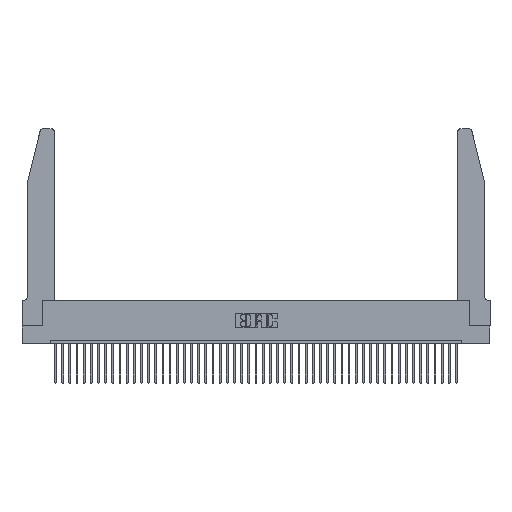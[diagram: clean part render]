
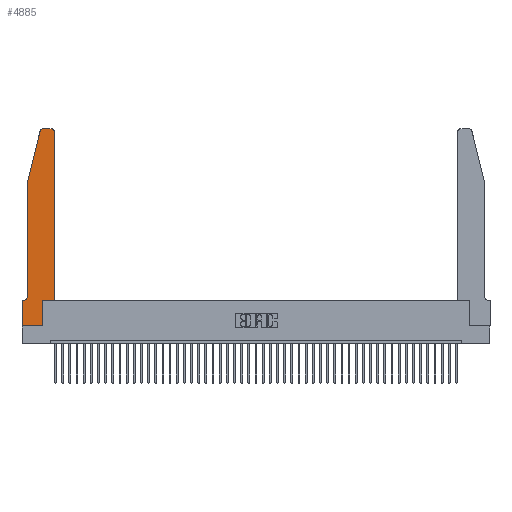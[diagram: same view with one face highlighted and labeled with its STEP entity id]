
A CAD part, top view. The second image highlights one B-rep face of the part: STEP entity #4885.
In plain terms, the highlighted planar face has unit normal (0, 0, 1).
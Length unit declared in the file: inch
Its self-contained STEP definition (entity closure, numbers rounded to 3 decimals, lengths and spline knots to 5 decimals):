
#571 = ORIENTED_EDGE ( 'NONE', *, *, #3788, .T. ) ;
#582 = CARTESIAN_POINT ( 'NONE',  ( 0.4205, 2.72, 0.37 ) ) ;
#734 = VECTOR ( 'NONE', #34522, 39.37008 ) ;
#787 = EDGE_CURVE ( 'NONE', #12762, #23518, #35287, .T. ) ;
#831 = EDGE_CURVE ( 'NONE', #11909, #4511, #42408, .T. ) ;
#1153 = CIRCLE ( 'NONE', #28801, 0.03 ) ;
#1297 = CARTESIAN_POINT ( 'NONE',  ( 0.0755, 0.35, 0.37 ) ) ;
#2896 = CARTESIAN_POINT ( 'NONE',  ( 0.25487, 2.72718, 0.37 ) ) ;
#3256 = LINE ( 'NONE', #25785, #9827 ) ;
#3788 = EDGE_CURVE ( 'NONE', #25622, #34251, #30043, .T. ) ;
#4511 = VERTEX_POINT ( 'NONE', #27140 ) ;
#4738 = EDGE_CURVE ( 'NONE', #8707, #5197, #35386, .T. ) ;
#4885 = ADVANCED_FACE ( 'NONE', ( #39185 ), #19686, .T. ) ;
#5061 = ORIENTED_EDGE ( 'NONE', *, *, #39481, .T. ) ;
#5080 = VERTEX_POINT ( 'NONE', #42720 ) ;
#5197 = VERTEX_POINT ( 'NONE', #16245 ) ;
#6794 = EDGE_CURVE ( 'NONE', #5080, #25622, #14798, .T. ) ;
#6840 = ORIENTED_EDGE ( 'NONE', *, *, #831, .T. ) ;
#8315 = CARTESIAN_POINT ( 'NONE',  ( 0.0055, 0.35, 0.37 ) ) ;
#8447 = ORIENTED_EDGE ( 'NONE', *, *, #43320, .T. ) ;
#8448 = EDGE_CURVE ( 'NONE', #5197, #29494, #24437, .T. ) ;
#8707 = VERTEX_POINT ( 'NONE', #33615 ) ;
#9535 = CIRCLE ( 'NONE', #19520, 0.07 ) ;
#9661 = ORIENTED_EDGE ( 'NONE', *, *, #6794, .T. ) ;
#9827 = VECTOR ( 'NONE', #18657, 39.37008 ) ;
#10448 = CARTESIAN_POINT ( 'NONE',  ( 0.284, 2.75, 0.37 ) ) ;
#11121 = EDGE_CURVE ( 'NONE', #4511, #43242, #42914, .T. ) ;
#11230 = VECTOR ( 'NONE', #39937, 39.37008 ) ;
#11909 = VERTEX_POINT ( 'NONE', #2896 ) ;
#12346 = VECTOR ( 'NONE', #30002, 39.37008 ) ;
#12762 = VERTEX_POINT ( 'NONE', #8315 ) ;
#12878 = DIRECTION ( 'NONE',  ( 0., 0., 1. ) ) ;
#14128 = AXIS2_PLACEMENT_3D ( 'NONE', #44157, #12878, #19218 ) ;
#14798 = LINE ( 'NONE', #44548, #27015 ) ;
#15009 = CARTESIAN_POINT ( 'NONE',  ( 0.0755, 2., 0.37 ) ) ;
#16004 = CARTESIAN_POINT ( 'NONE',  ( 0., 0.35, 0.37 ) ) ;
#16094 = CARTESIAN_POINT ( 'NONE',  ( 0.4505, 0.35, 0.37 ) ) ;
#16245 = CARTESIAN_POINT ( 'NONE',  ( 0.4205, 2.75, 0.37 ) ) ;
#16838 = ORIENTED_EDGE ( 'NONE', *, *, #32134, .T. ) ;
#17101 = DIRECTION ( 'NONE',  ( 0., 0., 1. ) ) ;
#17251 = DIRECTION ( 'NONE',  ( 0., 1., 0. ) ) ;
#17476 = CARTESIAN_POINT ( 'NONE',  ( 0.0055, 0.42, 0.37 ) ) ;
#18141 = EDGE_CURVE ( 'NONE', #23518, #27206, #3256, .T. ) ;
#18606 = ORIENTED_EDGE ( 'NONE', *, *, #11121, .T. ) ;
#18657 = DIRECTION ( 'NONE',  ( 0., -1., 0. ) ) ;
#18895 = EDGE_LOOP ( 'NONE', ( #34331, #5061, #6840, #18606, #8447, #29280, #25458, #39552, #9661, #571, #16838, #32084 ) ) ;
#19218 = DIRECTION ( 'NONE',  ( 1., 0., 0. ) ) ;
#19520 = AXIS2_PLACEMENT_3D ( 'NONE', #17476, #31684, #42531 ) ;
#19590 = CARTESIAN_POINT ( 'NONE',  ( 0.4505, 0.35, 0.37 ) ) ;
#19686 = PLANE ( 'NONE',  #14128 ) ;
#20071 = CARTESIAN_POINT ( 'NONE',  ( 0.2605, 2.75, 0.37 ) ) ;
#20966 = CARTESIAN_POINT ( 'NONE',  ( 0.284, 2.72, 0.37 ) ) ;
#21404 = CARTESIAN_POINT ( 'NONE',  ( 0., 0., 0.37 ) ) ;
#23472 = CARTESIAN_POINT ( 'NONE',  ( 0.0755, 2., 0.37 ) ) ;
#23518 = VERTEX_POINT ( 'NONE', #16004 ) ;
#23695 = CARTESIAN_POINT ( 'NONE',  ( 0.2865, 0.35, 0.37 ) ) ;
#24430 = DIRECTION ( 'NONE',  ( 1., 0., 0. ) ) ;
#24437 = LINE ( 'NONE', #20071, #734 ) ;
#25406 = DIRECTION ( 'NONE',  ( 1., 0., 0. ) ) ;
#25458 = ORIENTED_EDGE ( 'NONE', *, *, #18141, .T. ) ;
#25622 = VERTEX_POINT ( 'NONE', #23695 ) ;
#25785 = CARTESIAN_POINT ( 'NONE',  ( 0., 0., 0.37 ) ) ;
#27004 = DIRECTION ( 'NONE',  ( 0., -1., 0. ) ) ;
#27015 = VECTOR ( 'NONE', #17251, 39.37008 ) ;
#27140 = CARTESIAN_POINT ( 'NONE',  ( 0.0755, 2., 0.37 ) ) ;
#27206 = VERTEX_POINT ( 'NONE', #21404 ) ;
#28180 = VECTOR ( 'NONE', #40215, 39.37008 ) ;
#28801 = AXIS2_PLACEMENT_3D ( 'NONE', #20966, #17101, #45617 ) ;
#29081 = LINE ( 'NONE', #33995, #30192 ) ;
#29280 = ORIENTED_EDGE ( 'NONE', *, *, #787, .T. ) ;
#29494 = VERTEX_POINT ( 'NONE', #10448 ) ;
#29529 = CARTESIAN_POINT ( 'NONE',  ( 0.4505, 0.35, 0.37 ) ) ;
#29814 = AXIS2_PLACEMENT_3D ( 'NONE', #582, #39335, #25406 ) ;
#30002 = DIRECTION ( 'NONE',  ( 0., 1., 0. ) ) ;
#30043 = LINE ( 'NONE', #29529, #11230 ) ;
#30192 = VECTOR ( 'NONE', #24430, 39.37008 ) ;
#30878 = DIRECTION ( 'NONE',  ( -0.239, -0.971, 0. ) ) ;
#31684 = DIRECTION ( 'NONE',  ( 0., 0., -1. ) ) ;
#32084 = ORIENTED_EDGE ( 'NONE', *, *, #4738, .T. ) ;
#32134 = EDGE_CURVE ( 'NONE', #34251, #8707, #40986, .T. ) ;
#33088 = VECTOR ( 'NONE', #30878, 39.37008 ) ;
#33615 = CARTESIAN_POINT ( 'NONE',  ( 0.4505, 2.72, 0.37 ) ) ;
#33995 = CARTESIAN_POINT ( 'NONE',  ( 0., 0., 0.37 ) ) ;
#34251 = VERTEX_POINT ( 'NONE', #19590 ) ;
#34279 = CARTESIAN_POINT ( 'NONE',  ( 0.0755, 0.42, 0.37 ) ) ;
#34331 = ORIENTED_EDGE ( 'NONE', *, *, #8448, .T. ) ;
#34522 = DIRECTION ( 'NONE',  ( -1., 0., 0. ) ) ;
#35287 = LINE ( 'NONE', #1297, #28180 ) ;
#35386 = CIRCLE ( 'NONE', #29814, 0.03 ) ;
#39185 = FACE_OUTER_BOUND ( 'NONE', #18895, .T. ) ;
#39335 = DIRECTION ( 'NONE',  ( 0., 0., 1. ) ) ;
#39481 = EDGE_CURVE ( 'NONE', #29494, #11909, #1153, .T. ) ;
#39552 = ORIENTED_EDGE ( 'NONE', *, *, #41450, .T. ) ;
#39937 = DIRECTION ( 'NONE',  ( 1., 0., 0. ) ) ;
#40215 = DIRECTION ( 'NONE',  ( -1., 0., 0. ) ) ;
#40986 = LINE ( 'NONE', #16094, #12346 ) ;
#41450 = EDGE_CURVE ( 'NONE', #27206, #5080, #29081, .T. ) ;
#41842 = VECTOR ( 'NONE', #27004, 39.37008 ) ;
#42408 = LINE ( 'NONE', #23472, #33088 ) ;
#42531 = DIRECTION ( 'NONE',  ( -1., 0., 0. ) ) ;
#42720 = CARTESIAN_POINT ( 'NONE',  ( 0.2865, 0., 0.37 ) ) ;
#42914 = LINE ( 'NONE', #15009, #41842 ) ;
#43242 = VERTEX_POINT ( 'NONE', #34279 ) ;
#43320 = EDGE_CURVE ( 'NONE', #43242, #12762, #9535, .T. ) ;
#44157 = CARTESIAN_POINT ( 'NONE',  ( 0., 0.35, 0.37 ) ) ;
#44548 = CARTESIAN_POINT ( 'NONE',  ( 0.2865, 0.35, 0.37 ) ) ;
#45617 = DIRECTION ( 'NONE',  ( 1., 0., 0. ) ) ;
